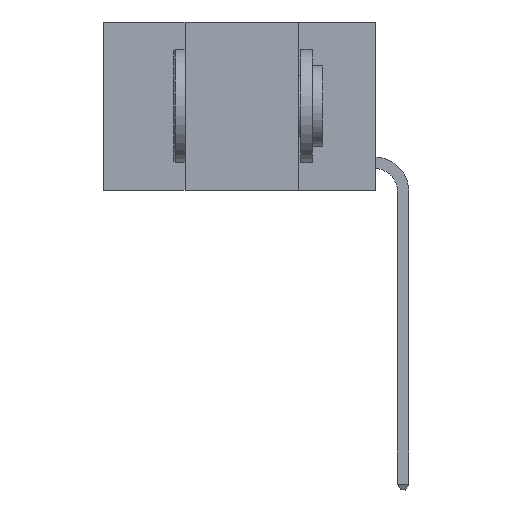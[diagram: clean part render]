
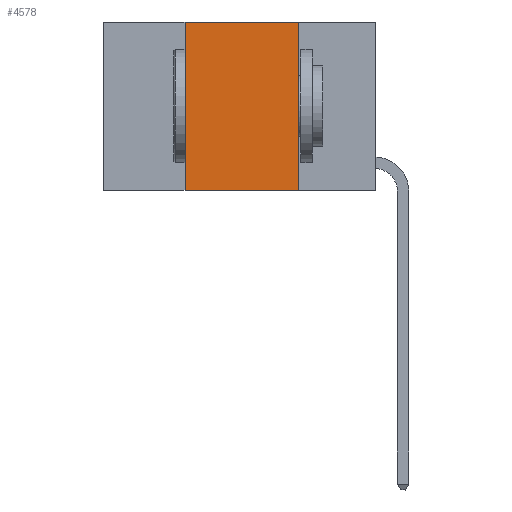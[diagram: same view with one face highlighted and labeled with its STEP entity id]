
A CAD part, left-side view. The second image highlights one B-rep face of the part: STEP entity #4578.
In plain terms, the highlighted planar face has unit normal (-1, 0, 0).
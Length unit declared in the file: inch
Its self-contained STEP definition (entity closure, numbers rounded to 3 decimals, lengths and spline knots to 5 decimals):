
#93 = VECTOR ( 'NONE', #1791, 39.37008 ) ;
#376 = LINE ( 'NONE', #15267, #16588 ) ;
#408 = CARTESIAN_POINT ( 'NONE',  ( 0., 0.42, 0. ) ) ;
#1175 = DIRECTION ( 'NONE',  ( 0., 0., -1. ) ) ;
#1791 = DIRECTION ( 'NONE',  ( 0., 0., 1. ) ) ;
#1972 = DIRECTION ( 'NONE',  ( 0., -1., 0. ) ) ;
#2796 = ORIENTED_EDGE ( 'NONE', *, *, #2854, .F. ) ;
#2854 = EDGE_CURVE ( 'NONE', #4405, #5567, #376, .T. ) ;
#3340 = DIRECTION ( 'NONE',  ( 0., -1., 0. ) ) ;
#3929 = AXIS2_PLACEMENT_3D ( 'NONE', #17132, #15850, #1175 ) ;
#4312 = EDGE_CURVE ( 'NONE', #20679, #14060, #4732, .T. ) ;
#4405 = VERTEX_POINT ( 'NONE', #9606 ) ;
#4578 = ADVANCED_FACE ( 'NONE', ( #18833 ), #19147, .F. ) ;
#4600 = VECTOR ( 'NONE', #3340, 39.37008 ) ;
#4732 = LINE ( 'NONE', #14805, #4600 ) ;
#5567 = VERTEX_POINT ( 'NONE', #13508 ) ;
#6358 = VECTOR ( 'NONE', #15250, 39.37008 ) ;
#7450 = ORIENTED_EDGE ( 'NONE', *, *, #4312, .T. ) ;
#8961 = ORIENTED_EDGE ( 'NONE', *, *, #20863, .F. ) ;
#9606 = CARTESIAN_POINT ( 'NONE',  ( 0., 0.42, 0. ) ) ;
#9886 = LINE ( 'NONE', #408, #93 ) ;
#10950 = EDGE_CURVE ( 'NONE', #20679, #4405, #9886, .T. ) ;
#11253 = CARTESIAN_POINT ( 'NONE',  ( 0., 0.17, -0.37 ) ) ;
#13508 = CARTESIAN_POINT ( 'NONE',  ( 0., 0.17, 0. ) ) ;
#13730 = CARTESIAN_POINT ( 'NONE',  ( 0., 0.17, 0. ) ) ;
#14060 = VERTEX_POINT ( 'NONE', #11253 ) ;
#14805 = CARTESIAN_POINT ( 'NONE',  ( 0., 0.6, -0.37 ) ) ;
#15250 = DIRECTION ( 'NONE',  ( 0., 0., -1. ) ) ;
#15267 = CARTESIAN_POINT ( 'NONE',  ( 0., 0.6, 0. ) ) ;
#15663 = LINE ( 'NONE', #13730, #6358 ) ;
#15841 = EDGE_LOOP ( 'NONE', ( #8961, #2796, #18074, #7450 ) ) ;
#15850 = DIRECTION ( 'NONE',  ( 1., 0., 0. ) ) ;
#16588 = VECTOR ( 'NONE', #1972, 39.37008 ) ;
#16731 = CARTESIAN_POINT ( 'NONE',  ( 0., 0.42, -0.37 ) ) ;
#17132 = CARTESIAN_POINT ( 'NONE',  ( 0., 0.6, 0. ) ) ;
#18074 = ORIENTED_EDGE ( 'NONE', *, *, #10950, .F. ) ;
#18833 = FACE_OUTER_BOUND ( 'NONE', #15841, .T. ) ;
#19147 = PLANE ( 'NONE',  #3929 ) ;
#20679 = VERTEX_POINT ( 'NONE', #16731 ) ;
#20863 = EDGE_CURVE ( 'NONE', #5567, #14060, #15663, .T. ) ;
